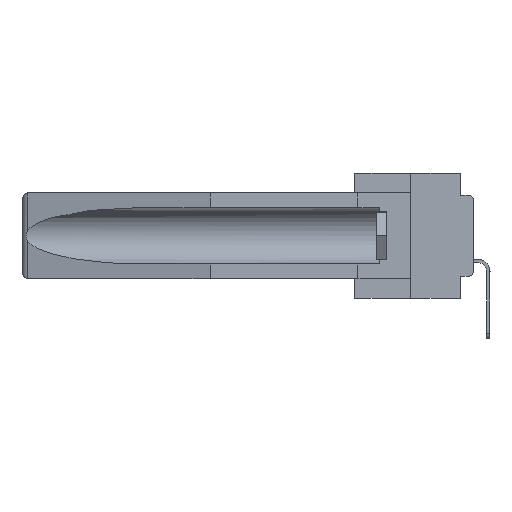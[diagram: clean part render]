
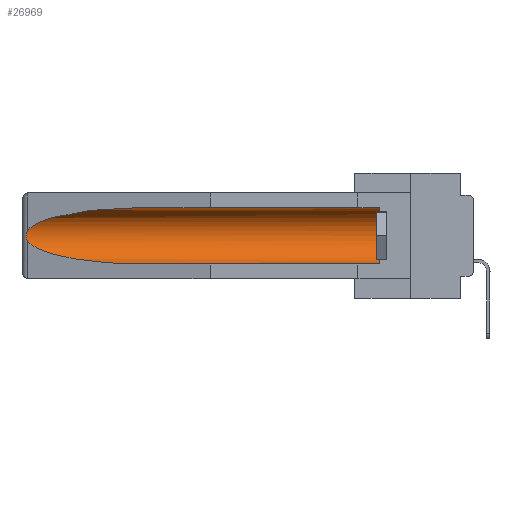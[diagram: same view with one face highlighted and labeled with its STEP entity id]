
A CAD part, left-side view. The second image highlights one B-rep face of the part: STEP entity #26969.
In plain terms, the highlighted cylindrical face has radius 2.857 mm (diameter 5.715 mm), a partial arc.
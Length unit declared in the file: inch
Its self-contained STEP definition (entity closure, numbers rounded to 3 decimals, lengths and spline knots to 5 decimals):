
#146 =( BOUNDED_CURVE ( )  B_SPLINE_CURVE ( 3, ( #15503, #24215, #15795, #2196 ),
 .UNSPECIFIED., .F., .T. ) 
 B_SPLINE_CURVE_WITH_KNOTS ( ( 4, 4 ),
 ( 4.71239, 6.08839 ),
 .UNSPECIFIED. ) 
 CURVE ( )  GEOMETRIC_REPRESENTATION_ITEM ( )  RATIONAL_B_SPLINE_CURVE ( ( 1., 0.848, 0.848, 1. ) ) 
 REPRESENTATION_ITEM ( '' )  );
#311 =( BOUNDED_CURVE ( )  B_SPLINE_CURVE ( 3, ( #3801, #2078, #6342, #28268 ),
 .UNSPECIFIED., .F., .T. ) 
 B_SPLINE_CURVE_WITH_KNOTS ( ( 4, 4 ),
 ( 0.1948, 1.5708 ),
 .UNSPECIFIED. ) 
 CURVE ( )  GEOMETRIC_REPRESENTATION_ITEM ( )  RATIONAL_B_SPLINE_CURVE ( ( 1., 0.848, 0.848, 1. ) ) 
 REPRESENTATION_ITEM ( '' )  );
#606 = AXIS2_PLACEMENT_3D ( 'NONE', #21618, #2029, #10748 ) ;
#1192 = AXIS2_PLACEMENT_3D ( 'NONE', #13383, #13531, #9054 ) ;
#1904 = VERTEX_POINT ( 'NONE', #16907 ) ;
#2029 = DIRECTION ( 'NONE',  ( 0., -1., 0. ) ) ;
#2078 = CARTESIAN_POINT ( 'NONE',  ( 0.25451, 1.48313, -0.24835 ) ) ;
#2196 = CARTESIAN_POINT ( 'NONE',  ( 0.26537, 1.52718, -0.14972 ) ) ;
#2900 = VERTEX_POINT ( 'NONE', #11189 ) ;
#3067 = CARTESIAN_POINT ( 'NONE',  ( 0.2673, 1.53269, -0.17917 ) ) ;
#3801 = CARTESIAN_POINT ( 'NONE',  ( 0.26537, 1.52718, -0.19328 ) ) ;
#4019 = VERTEX_POINT ( 'NONE', #27028 ) ;
#4266 = EDGE_CURVE ( 'NONE', #5534, #16022, #10950, .T. ) ;
#4310 = EDGE_CURVE ( 'NONE', #1904, #4019, #5087, .T. ) ;
#4633 = FACE_OUTER_BOUND ( 'NONE', #25889, .T. ) ;
#4927 = CARTESIAN_POINT ( 'NONE',  ( 0.26654, 1.53092, -0.15636 ) ) ;
#5087 = LINE ( 'NONE', #22401, #13633 ) ;
#5205 = CARTESIAN_POINT ( 'NONE',  ( 0.26537, 1.52718, -0.19328 ) ) ;
#5248 = CARTESIAN_POINT ( 'NONE',  ( 0.26537, 1.52718, -0.19328 ) ) ;
#5534 = VERTEX_POINT ( 'NONE', #26152 ) ;
#6342 = CARTESIAN_POINT ( 'NONE',  ( 0.21114, 1.30732, -0.284 ) ) ;
#6650 = ORIENTED_EDGE ( 'NONE', *, *, #4266, .T. ) ;
#6959 = VERTEX_POINT ( 'NONE', #5248 ) ;
#7202 = CARTESIAN_POINT ( 'NONE',  ( 0.26597, 1.5296, -0.19026 ) ) ;
#8262 = ORIENTED_EDGE ( 'NONE', *, *, #18720, .T. ) ;
#8507 = EDGE_CURVE ( 'NONE', #16022, #2900, #146, .T. ) ;
#9052 = CARTESIAN_POINT ( 'NONE',  ( 0.26537, 1.52718, -0.14972 ) ) ;
#9054 = DIRECTION ( 'NONE',  ( 0., 0., 1. ) ) ;
#9892 = ORIENTED_EDGE ( 'NONE', *, *, #13207, .T. ) ;
#10147 = EDGE_CURVE ( 'NONE', #1904, #5534, #21609, .T. ) ;
#10348 = B_SPLINE_CURVE_WITH_KNOTS ( 'NONE', 3,
 ( #9052, #15667, #4927, #20389, #16095, #15952, #3067, #13529, #7202, #5205 ),
 .UNSPECIFIED., .F., .F.,
 ( 4, 2, 2, 2, 4 ),
 ( 0., 0.00029, 0.00058, 0.00087, 0.00117 ),
 .UNSPECIFIED. ) ;
#10748 = DIRECTION ( 'NONE',  ( 0., 0., 1. ) ) ;
#10929 = CYLINDRICAL_SURFACE ( 'NONE', #1192, 0.1125 ) ;
#10950 = LINE ( 'NONE', #11529, #14085 ) ;
#11189 = CARTESIAN_POINT ( 'NONE',  ( 0.26537, 1.52718, -0.14972 ) ) ;
#11529 = CARTESIAN_POINT ( 'NONE',  ( 0.155, -0.30754, -0.059 ) ) ;
#13207 = EDGE_CURVE ( 'NONE', #2900, #6959, #10348, .T. ) ;
#13383 = CARTESIAN_POINT ( 'NONE',  ( 0.155, -0.30754, -0.1715 ) ) ;
#13529 = CARTESIAN_POINT ( 'NONE',  ( 0.26655, 1.53094, -0.18657 ) ) ;
#13531 = DIRECTION ( 'NONE',  ( 0., 1., 0. ) ) ;
#13633 = VECTOR ( 'NONE', #26854, 39.37008 ) ;
#14085 = VECTOR ( 'NONE', #19848, 39.37008 ) ;
#15503 = CARTESIAN_POINT ( 'NONE',  ( 0.155, 1.07973, -0.059 ) ) ;
#15667 = CARTESIAN_POINT ( 'NONE',  ( 0.26597, 1.52961, -0.15275 ) ) ;
#15795 = CARTESIAN_POINT ( 'NONE',  ( 0.25451, 1.48313, -0.09465 ) ) ;
#15952 = CARTESIAN_POINT ( 'NONE',  ( 0.2675, 1.53308, -0.17534 ) ) ;
#16022 = VERTEX_POINT ( 'NONE', #19140 ) ;
#16095 = CARTESIAN_POINT ( 'NONE',  ( 0.2675, 1.53308, -0.16763 ) ) ;
#16907 = CARTESIAN_POINT ( 'NONE',  ( 0.155, 0.126, -0.284 ) ) ;
#18720 = EDGE_CURVE ( 'NONE', #6959, #4019, #311, .T. ) ;
#19140 = CARTESIAN_POINT ( 'NONE',  ( 0.155, 1.07973, -0.059 ) ) ;
#19848 = DIRECTION ( 'NONE',  ( 0., 1., 0. ) ) ;
#20389 = CARTESIAN_POINT ( 'NONE',  ( 0.2673, 1.5327, -0.16383 ) ) ;
#21609 = CIRCLE ( 'NONE', #606, 0.1125 ) ;
#21618 = CARTESIAN_POINT ( 'NONE',  ( 0.155, 0.126, -0.1715 ) ) ;
#22292 = ORIENTED_EDGE ( 'NONE', *, *, #4310, .F. ) ;
#22401 = CARTESIAN_POINT ( 'NONE',  ( 0.155, -0.30754, -0.284 ) ) ;
#23448 = ORIENTED_EDGE ( 'NONE', *, *, #10147, .T. ) ;
#24215 = CARTESIAN_POINT ( 'NONE',  ( 0.21114, 1.30732, -0.059 ) ) ;
#25889 = EDGE_LOOP ( 'NONE', ( #26380, #9892, #8262, #22292, #23448, #6650 ) ) ;
#26152 = CARTESIAN_POINT ( 'NONE',  ( 0.155, 0.126, -0.059 ) ) ;
#26380 = ORIENTED_EDGE ( 'NONE', *, *, #8507, .T. ) ;
#26854 = DIRECTION ( 'NONE',  ( 0., 1., 0. ) ) ;
#26969 = ADVANCED_FACE ( 'NONE', ( #4633 ), #10929, .F. ) ;
#27028 = CARTESIAN_POINT ( 'NONE',  ( 0.155, 1.07973, -0.284 ) ) ;
#28268 = CARTESIAN_POINT ( 'NONE',  ( 0.155, 1.07973, -0.284 ) ) ;
